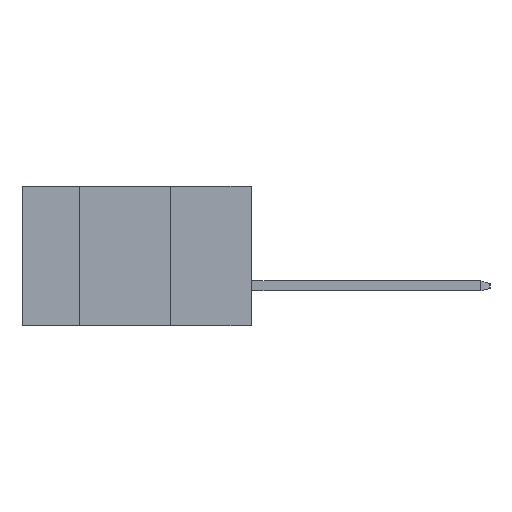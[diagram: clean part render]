
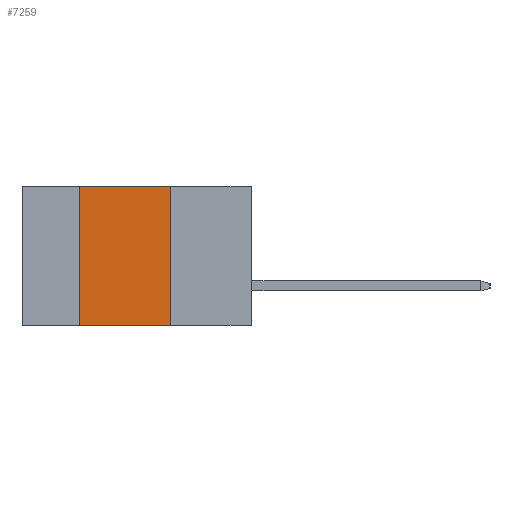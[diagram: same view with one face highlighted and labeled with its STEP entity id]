
A CAD part, left-side view. The second image highlights one B-rep face of the part: STEP entity #7259.
In plain terms, the highlighted planar face has unit normal (-1, 0, 0).
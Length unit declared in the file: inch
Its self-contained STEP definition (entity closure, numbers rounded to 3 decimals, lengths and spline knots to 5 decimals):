
#173 = CARTESIAN_POINT ( 'NONE',  ( 0., 0.72, 0. ) ) ;
#319 = CARTESIAN_POINT ( 'NONE',  ( 0., 0.254, -0.437 ) ) ;
#657 = CARTESIAN_POINT ( 'NONE',  ( 0., 0.54, -0.437 ) ) ;
#796 = LINE ( 'NONE', #173, #5860 ) ;
#1330 = DIRECTION ( 'NONE',  ( 1., 0., 0. ) ) ;
#1463 = VECTOR ( 'NONE', #6347, 39.37008 ) ;
#1491 = LINE ( 'NONE', #4077, #1463 ) ;
#2106 = EDGE_CURVE ( 'NONE', #4361, #9883, #2363, .T. ) ;
#2363 = LINE ( 'NONE', #5497, #3170 ) ;
#2379 = PLANE ( 'NONE',  #3932 ) ;
#2771 = ORIENTED_EDGE ( 'NONE', *, *, #6322, .F. ) ;
#2888 = DIRECTION ( 'NONE',  ( 0., 0., 1. ) ) ;
#3170 = VECTOR ( 'NONE', #4057, 39.37008 ) ;
#3434 = ORIENTED_EDGE ( 'NONE', *, *, #2106, .T. ) ;
#3676 = EDGE_LOOP ( 'NONE', ( #9974, #4524, #2771, #3434 ) ) ;
#3932 = AXIS2_PLACEMENT_3D ( 'NONE', #8409, #1330, #10073 ) ;
#4057 = DIRECTION ( 'NONE',  ( 0., -1., 0. ) ) ;
#4077 = CARTESIAN_POINT ( 'NONE',  ( 0., 0.254, -0.437 ) ) ;
#4361 = VERTEX_POINT ( 'NONE', #7433 ) ;
#4524 = ORIENTED_EDGE ( 'NONE', *, *, #4994, .F. ) ;
#4994 = EDGE_CURVE ( 'NONE', #6530, #9382, #796, .T. ) ;
#5497 = CARTESIAN_POINT ( 'NONE',  ( 0., 0.72, -0.437 ) ) ;
#5860 = VECTOR ( 'NONE', #6468, 39.37008 ) ;
#6322 = EDGE_CURVE ( 'NONE', #4361, #6530, #8392, .T. ) ;
#6347 = DIRECTION ( 'NONE',  ( 0., 0., -1. ) ) ;
#6468 = DIRECTION ( 'NONE',  ( 0., -1., 0. ) ) ;
#6472 = CARTESIAN_POINT ( 'NONE',  ( 0., 0.254, 0. ) ) ;
#6530 = VERTEX_POINT ( 'NONE', #8603 ) ;
#6896 = FACE_OUTER_BOUND ( 'NONE', #3676, .T. ) ;
#7259 = ADVANCED_FACE ( 'NONE', ( #6896 ), #2379, .F. ) ;
#7433 = CARTESIAN_POINT ( 'NONE',  ( 0., 0.54, -0.437 ) ) ;
#8392 = LINE ( 'NONE', #657, #9690 ) ;
#8409 = CARTESIAN_POINT ( 'NONE',  ( 0., 0.72, 0. ) ) ;
#8603 = CARTESIAN_POINT ( 'NONE',  ( 0., 0.54, 0. ) ) ;
#9382 = VERTEX_POINT ( 'NONE', #6472 ) ;
#9690 = VECTOR ( 'NONE', #2888, 39.37008 ) ;
#9883 = VERTEX_POINT ( 'NONE', #319 ) ;
#9974 = ORIENTED_EDGE ( 'NONE', *, *, #10108, .F. ) ;
#10073 = DIRECTION ( 'NONE',  ( 0., 0., -1. ) ) ;
#10108 = EDGE_CURVE ( 'NONE', #9382, #9883, #1491, .T. ) ;
